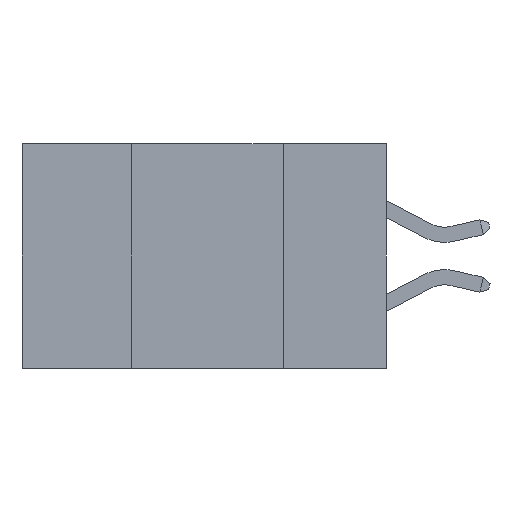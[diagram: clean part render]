
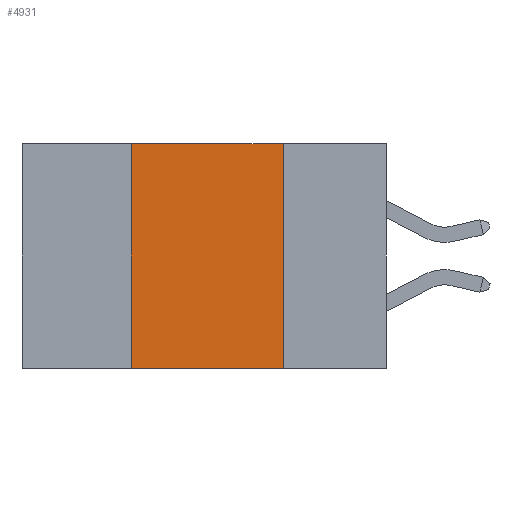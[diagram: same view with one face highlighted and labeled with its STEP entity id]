
A CAD part, left-side view. The second image highlights one B-rep face of the part: STEP entity #4931.
In plain terms, the highlighted planar face has unit normal (-1, 0, 0).
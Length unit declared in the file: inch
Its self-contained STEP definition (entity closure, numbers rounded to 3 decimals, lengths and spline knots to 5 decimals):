
#123 = AXIS2_PLACEMENT_3D ( 'NONE', #172, #989, #7405 ) ;
#172 = CARTESIAN_POINT ( 'NONE',  ( 0., 0.6, 0. ) ) ;
#571 = ORIENTED_EDGE ( 'NONE', *, *, #9508, .F. ) ;
#572 = LINE ( 'NONE', #10400, #4076 ) ;
#989 = DIRECTION ( 'NONE',  ( 1., 0., 0. ) ) ;
#1322 = VECTOR ( 'NONE', #2232, 39.37008 ) ;
#2232 = DIRECTION ( 'NONE',  ( 0., 0., -1. ) ) ;
#2653 = DIRECTION ( 'NONE',  ( 0., -1., 0. ) ) ;
#3026 = LINE ( 'NONE', #4325, #3660 ) ;
#3192 = CARTESIAN_POINT ( 'NONE',  ( 0., 0.42, -0.37 ) ) ;
#3225 = ORIENTED_EDGE ( 'NONE', *, *, #6953, .F. ) ;
#3251 = CARTESIAN_POINT ( 'NONE',  ( 0., 0.17, -0.37 ) ) ;
#3376 = PLANE ( 'NONE',  #123 ) ;
#3660 = VECTOR ( 'NONE', #9991, 39.37008 ) ;
#4076 = VECTOR ( 'NONE', #10401, 39.37008 ) ;
#4228 = VERTEX_POINT ( 'NONE', #6330 ) ;
#4256 = VERTEX_POINT ( 'NONE', #8004 ) ;
#4325 = CARTESIAN_POINT ( 'NONE',  ( 0., 0.42, -0.37 ) ) ;
#4520 = VERTEX_POINT ( 'NONE', #3192 ) ;
#4796 = EDGE_LOOP ( 'NONE', ( #3225, #10126, #571, #8893 ) ) ;
#4893 = VECTOR ( 'NONE', #2653, 39.37008 ) ;
#4931 = ADVANCED_FACE ( 'NONE', ( #6275 ), #3376, .F. ) ;
#5104 = CARTESIAN_POINT ( 'NONE',  ( 0., 0.6, -0.37 ) ) ;
#5298 = EDGE_CURVE ( 'NONE', #4520, #6799, #6393, .T. ) ;
#6275 = FACE_OUTER_BOUND ( 'NONE', #4796, .T. ) ;
#6330 = CARTESIAN_POINT ( 'NONE',  ( 0., 0.42, 0. ) ) ;
#6393 = LINE ( 'NONE', #5104, #4893 ) ;
#6649 = EDGE_CURVE ( 'NONE', #4228, #4256, #572, .T. ) ;
#6799 = VERTEX_POINT ( 'NONE', #3251 ) ;
#6953 = EDGE_CURVE ( 'NONE', #4256, #6799, #9138, .T. ) ;
#7405 = DIRECTION ( 'NONE',  ( 0., 0., -1. ) ) ;
#8004 = CARTESIAN_POINT ( 'NONE',  ( 0., 0.17, 0. ) ) ;
#8630 = CARTESIAN_POINT ( 'NONE',  ( 0., 0.17, -0.37 ) ) ;
#8893 = ORIENTED_EDGE ( 'NONE', *, *, #5298, .T. ) ;
#9138 = LINE ( 'NONE', #8630, #1322 ) ;
#9508 = EDGE_CURVE ( 'NONE', #4520, #4228, #3026, .T. ) ;
#9991 = DIRECTION ( 'NONE',  ( 0., 0., 1. ) ) ;
#10126 = ORIENTED_EDGE ( 'NONE', *, *, #6649, .F. ) ;
#10400 = CARTESIAN_POINT ( 'NONE',  ( 0., 0.6, 0. ) ) ;
#10401 = DIRECTION ( 'NONE',  ( 0., -1., 0. ) ) ;
